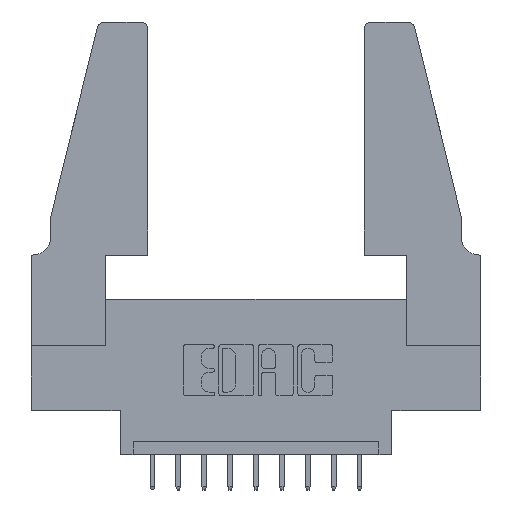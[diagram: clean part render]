
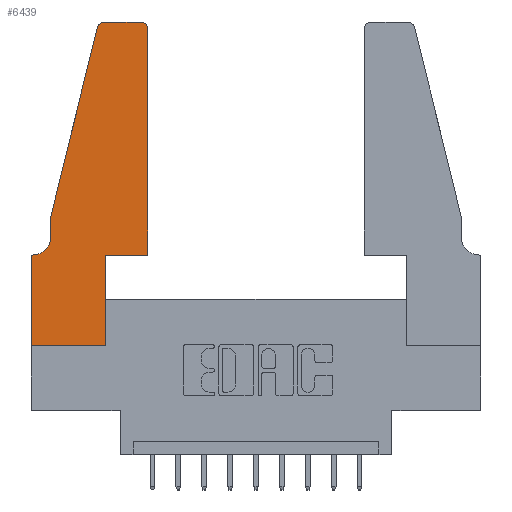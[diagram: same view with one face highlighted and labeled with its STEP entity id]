
A CAD part, top view. The second image highlights one B-rep face of the part: STEP entity #6439.
In plain terms, the highlighted planar face has unit normal (0, 0, 1).
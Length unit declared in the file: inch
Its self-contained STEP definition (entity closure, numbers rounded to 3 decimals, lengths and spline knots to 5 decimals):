
#96 = CARTESIAN_POINT ( 'NONE',  ( 0.2865, 0.35, 0.37 ) ) ;
#166 = VERTEX_POINT ( 'NONE', #11644 ) ;
#226 = LINE ( 'NONE', #4501, #6169 ) ;
#478 = DIRECTION ( 'NONE',  ( 1., 0., 0. ) ) ;
#571 = VERTEX_POINT ( 'NONE', #5346 ) ;
#887 = CIRCLE ( 'NONE', #3963, 0.07 ) ;
#1112 = FACE_OUTER_BOUND ( 'NONE', #9981, .T. ) ;
#1203 = EDGE_CURVE ( 'NONE', #13068, #12920, #887, .T. ) ;
#1371 = CARTESIAN_POINT ( 'NONE',  ( 0.4505, 0.35, 0.37 ) ) ;
#1432 = CARTESIAN_POINT ( 'NONE',  ( 0., 0., 0.37 ) ) ;
#1444 = CARTESIAN_POINT ( 'NONE',  ( 0.25487, 1.22718, 0.37 ) ) ;
#1481 = VECTOR ( 'NONE', #2506, 39.37008 ) ;
#1595 = CARTESIAN_POINT ( 'NONE',  ( 0.4505, 1.22, 0.37 ) ) ;
#1840 = DIRECTION ( 'NONE',  ( 1., 0., 0. ) ) ;
#1984 = EDGE_CURVE ( 'NONE', #8059, #12808, #11181, .T. ) ;
#2097 = DIRECTION ( 'NONE',  ( 0., 1., 0. ) ) ;
#2221 = DIRECTION ( 'NONE',  ( 0., 0., 1. ) ) ;
#2275 = ORIENTED_EDGE ( 'NONE', *, *, #8120, .T. ) ;
#2331 = EDGE_CURVE ( 'NONE', #12920, #11694, #7760, .T. ) ;
#2339 = ORIENTED_EDGE ( 'NONE', *, *, #8171, .T. ) ;
#2417 = CARTESIAN_POINT ( 'NONE',  ( 0.2865, 0., 0.37 ) ) ;
#2470 = DIRECTION ( 'NONE',  ( 0., 0., 1. ) ) ;
#2506 = DIRECTION ( 'NONE',  ( -1., 0., 0. ) ) ;
#2686 = CARTESIAN_POINT ( 'NONE',  ( 0.0755, 0.5, 0.37 ) ) ;
#3167 = ORIENTED_EDGE ( 'NONE', *, *, #11348, .T. ) ;
#3169 = VECTOR ( 'NONE', #2097, 39.37008 ) ;
#3856 = DIRECTION ( 'NONE',  ( -0.239, -0.971, 0. ) ) ;
#3890 = ORIENTED_EDGE ( 'NONE', *, *, #1203, .T. ) ;
#3963 = AXIS2_PLACEMENT_3D ( 'NONE', #10460, #13465, #8399 ) ;
#4010 = CARTESIAN_POINT ( 'NONE',  ( 0.284, 1.25, 0.37 ) ) ;
#4215 = PLANE ( 'NONE',  #10816 ) ;
#4386 = CARTESIAN_POINT ( 'NONE',  ( 0.0755, 0.5, 0.37 ) ) ;
#4458 = EDGE_CURVE ( 'NONE', #12808, #5354, #13141, .T. ) ;
#4465 = CIRCLE ( 'NONE', #11487, 0.03 ) ;
#4501 = CARTESIAN_POINT ( 'NONE',  ( 0.4505, 0.35, 0.37 ) ) ;
#4857 = EDGE_CURVE ( 'NONE', #571, #12206, #226, .T. ) ;
#4955 = DIRECTION ( 'NONE',  ( 1., 0., 0. ) ) ;
#5139 = CARTESIAN_POINT ( 'NONE',  ( 0.284, 1.22, 0.37 ) ) ;
#5306 = VECTOR ( 'NONE', #4955, 39.37008 ) ;
#5319 = ORIENTED_EDGE ( 'NONE', *, *, #10894, .T. ) ;
#5346 = CARTESIAN_POINT ( 'NONE',  ( 0.2865, 0.35, 0.37 ) ) ;
#5354 = VERTEX_POINT ( 'NONE', #1444 ) ;
#5632 = LINE ( 'NONE', #1432, #11708 ) ;
#5964 = DIRECTION ( 'NONE',  ( -1., 0., 0. ) ) ;
#5975 = ORIENTED_EDGE ( 'NONE', *, *, #2331, .T. ) ;
#5995 = CARTESIAN_POINT ( 'NONE',  ( 0., 0., 0.37 ) ) ;
#6169 = VECTOR ( 'NONE', #8772, 39.37008 ) ;
#6439 = ADVANCED_FACE ( 'NONE', ( #1112 ), #4215, .T. ) ;
#6506 = CARTESIAN_POINT ( 'NONE',  ( 0.0755, 0.42, 0.37 ) ) ;
#6514 = VERTEX_POINT ( 'NONE', #2417 ) ;
#6618 = CARTESIAN_POINT ( 'NONE',  ( 0.4205, 1.22, 0.37 ) ) ;
#6648 = VECTOR ( 'NONE', #11733, 39.37008 ) ;
#6652 = CARTESIAN_POINT ( 'NONE',  ( 0.0755, 0.35, 0.37 ) ) ;
#6737 = EDGE_CURVE ( 'NONE', #10504, #6514, #11207, .T. ) ;
#7255 = AXIS2_PLACEMENT_3D ( 'NONE', #5139, #9148, #1840 ) ;
#7296 = LINE ( 'NONE', #4386, #6648 ) ;
#7518 = ORIENTED_EDGE ( 'NONE', *, *, #6737, .T. ) ;
#7760 = LINE ( 'NONE', #6652, #1481 ) ;
#8059 = VERTEX_POINT ( 'NONE', #9498 ) ;
#8120 = EDGE_CURVE ( 'NONE', #11694, #10504, #5632, .T. ) ;
#8171 = EDGE_CURVE ( 'NONE', #12158, #8059, #4465, .T. ) ;
#8399 = DIRECTION ( 'NONE',  ( -1., 0., 0. ) ) ;
#8595 = EDGE_CURVE ( 'NONE', #166, #13068, #7296, .T. ) ;
#8693 = VECTOR ( 'NONE', #9265, 39.37008 ) ;
#8772 = DIRECTION ( 'NONE',  ( 1., 0., 0. ) ) ;
#8854 = ORIENTED_EDGE ( 'NONE', *, *, #4458, .T. ) ;
#9072 = CARTESIAN_POINT ( 'NONE',  ( 0.2605, 1.25, 0.37 ) ) ;
#9112 = VECTOR ( 'NONE', #3856, 39.37008 ) ;
#9148 = DIRECTION ( 'NONE',  ( 0., 0., 1. ) ) ;
#9265 = DIRECTION ( 'NONE',  ( 0., 1., 0. ) ) ;
#9498 = CARTESIAN_POINT ( 'NONE',  ( 0.4205, 1.25, 0.37 ) ) ;
#9654 = VECTOR ( 'NONE', #5964, 39.37008 ) ;
#9901 = ORIENTED_EDGE ( 'NONE', *, *, #1984, .T. ) ;
#9981 = EDGE_LOOP ( 'NONE', ( #9901, #8854, #5319, #11434, #3890, #5975, #2275, #7518, #13106, #10944, #3167, #2339 ) ) ;
#10460 = CARTESIAN_POINT ( 'NONE',  ( 0.0055, 0.42, 0.37 ) ) ;
#10504 = VERTEX_POINT ( 'NONE', #11917 ) ;
#10816 = AXIS2_PLACEMENT_3D ( 'NONE', #11633, #2221, #478 ) ;
#10818 = LINE ( 'NONE', #1371, #8693 ) ;
#10894 = EDGE_CURVE ( 'NONE', #5354, #166, #12933, .T. ) ;
#10944 = ORIENTED_EDGE ( 'NONE', *, *, #4857, .T. ) ;
#10979 = CARTESIAN_POINT ( 'NONE',  ( 0., 0.35, 0.37 ) ) ;
#11181 = LINE ( 'NONE', #9072, #9654 ) ;
#11207 = LINE ( 'NONE', #5995, #5306 ) ;
#11348 = EDGE_CURVE ( 'NONE', #12206, #12158, #10818, .T. ) ;
#11434 = ORIENTED_EDGE ( 'NONE', *, *, #8595, .T. ) ;
#11487 = AXIS2_PLACEMENT_3D ( 'NONE', #6618, #2470, #11881 ) ;
#11633 = CARTESIAN_POINT ( 'NONE',  ( 0., 0.35, 0.37 ) ) ;
#11644 = CARTESIAN_POINT ( 'NONE',  ( 0.0755, 0.5, 0.37 ) ) ;
#11673 = EDGE_CURVE ( 'NONE', #6514, #571, #12541, .T. ) ;
#11694 = VERTEX_POINT ( 'NONE', #10979 ) ;
#11708 = VECTOR ( 'NONE', #12977, 39.37008 ) ;
#11733 = DIRECTION ( 'NONE',  ( 0., -1., 0. ) ) ;
#11881 = DIRECTION ( 'NONE',  ( 1., 0., 0. ) ) ;
#11917 = CARTESIAN_POINT ( 'NONE',  ( 0., 0., 0.37 ) ) ;
#12158 = VERTEX_POINT ( 'NONE', #1595 ) ;
#12206 = VERTEX_POINT ( 'NONE', #13063 ) ;
#12541 = LINE ( 'NONE', #96, #3169 ) ;
#12808 = VERTEX_POINT ( 'NONE', #4010 ) ;
#12920 = VERTEX_POINT ( 'NONE', #13278 ) ;
#12933 = LINE ( 'NONE', #2686, #9112 ) ;
#12977 = DIRECTION ( 'NONE',  ( 0., -1., 0. ) ) ;
#13063 = CARTESIAN_POINT ( 'NONE',  ( 0.4505, 0.35, 0.37 ) ) ;
#13068 = VERTEX_POINT ( 'NONE', #6506 ) ;
#13106 = ORIENTED_EDGE ( 'NONE', *, *, #11673, .T. ) ;
#13141 = CIRCLE ( 'NONE', #7255, 0.03 ) ;
#13278 = CARTESIAN_POINT ( 'NONE',  ( 0.0055, 0.35, 0.37 ) ) ;
#13465 = DIRECTION ( 'NONE',  ( 0., 0., -1. ) ) ;
